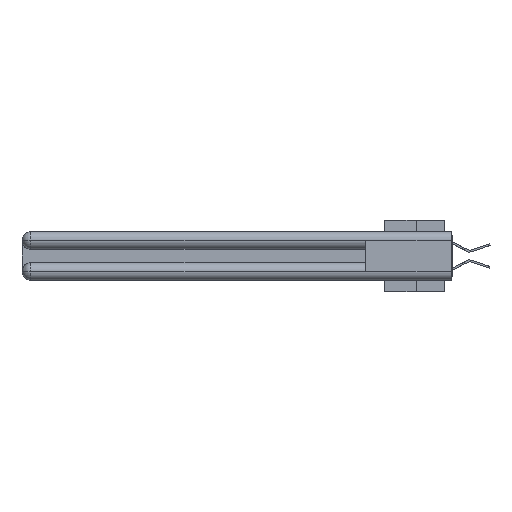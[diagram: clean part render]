
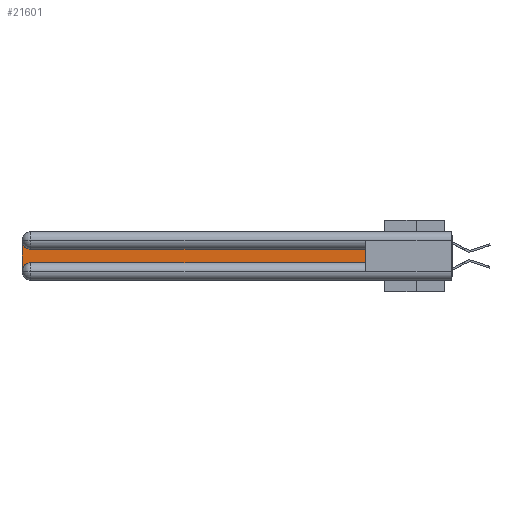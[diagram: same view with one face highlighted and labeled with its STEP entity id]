
A CAD part, left-side view. The second image highlights one B-rep face of the part: STEP entity #21601.
In plain terms, the highlighted planar face has unit normal (-1, 0, 0).
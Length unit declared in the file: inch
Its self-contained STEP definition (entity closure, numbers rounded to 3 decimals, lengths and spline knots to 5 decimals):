
#129 = VERTEX_POINT ( 'NONE', #13830 ) ;
#345 = AXIS2_PLACEMENT_3D ( 'NONE', #7179, #28323, #2479 ) ;
#801 = DIRECTION ( 'NONE',  ( 0., 1., 0. ) ) ;
#1193 = CIRCLE ( 'NONE', #16820, 0.06 ) ;
#2479 = DIRECTION ( 'NONE',  ( 0., 0., -1. ) ) ;
#4524 = DIRECTION ( 'NONE',  ( 0., -1., 0. ) ) ;
#5343 = CARTESIAN_POINT ( 'NONE',  ( 0.075, 0.6, -0.1225 ) ) ;
#5709 = CARTESIAN_POINT ( 'NONE',  ( 0.075, 2.94, -0.2775 ) ) ;
#5713 = EDGE_CURVE ( 'NONE', #21550, #12105, #23670, .T. ) ;
#5931 = CIRCLE ( 'NONE', #30431, 0.06 ) ;
#6310 = ORIENTED_EDGE ( 'NONE', *, *, #10745, .T. ) ;
#6891 = DIRECTION ( 'NONE',  ( 1., 0., 0. ) ) ;
#7179 = CARTESIAN_POINT ( 'NONE',  ( 0.075, 3., -0.1225 ) ) ;
#9151 = DIRECTION ( 'NONE',  ( 0., 0., -1. ) ) ;
#10745 = EDGE_CURVE ( 'NONE', #11620, #17671, #23314, .T. ) ;
#11353 = CARTESIAN_POINT ( 'NONE',  ( 0.075, 2.94, -0.0625 ) ) ;
#11408 = VECTOR ( 'NONE', #4524, 39.37008 ) ;
#11620 = VERTEX_POINT ( 'NONE', #21073 ) ;
#12105 = VERTEX_POINT ( 'NONE', #15975 ) ;
#12313 = CARTESIAN_POINT ( 'NONE',  ( 0.075, 2.94, -0.1225 ) ) ;
#12530 = CARTESIAN_POINT ( 'NONE',  ( 0.075, 3., -0.2775 ) ) ;
#13043 = DIRECTION ( 'NONE',  ( 1., 0., 0. ) ) ;
#13055 = ORIENTED_EDGE ( 'NONE', *, *, #21988, .T. ) ;
#13830 = CARTESIAN_POINT ( 'NONE',  ( 0.075, 2.94, -0.2175 ) ) ;
#14264 = VERTEX_POINT ( 'NONE', #12313 ) ;
#14452 = CARTESIAN_POINT ( 'NONE',  ( 0.075, 0.6, -0.2175 ) ) ;
#15285 = ORIENTED_EDGE ( 'NONE', *, *, #29850, .T. ) ;
#15975 = CARTESIAN_POINT ( 'NONE',  ( 0.075, 0.6, -0.1225 ) ) ;
#16073 = CARTESIAN_POINT ( 'NONE',  ( 0.075, 0.6, -0.2175 ) ) ;
#16195 = LINE ( 'NONE', #14452, #11408 ) ;
#16552 = EDGE_LOOP ( 'NONE', ( #30233, #16837, #6310, #13055, #15285, #23141 ) ) ;
#16721 = DIRECTION ( 'NONE',  ( 0., 0., -1. ) ) ;
#16820 = AXIS2_PLACEMENT_3D ( 'NONE', #5709, #13043, #17515 ) ;
#16837 = ORIENTED_EDGE ( 'NONE', *, *, #17209, .T. ) ;
#17209 = EDGE_CURVE ( 'NONE', #14264, #11620, #5931, .T. ) ;
#17515 = DIRECTION ( 'NONE',  ( 0., 0., -1. ) ) ;
#17671 = VERTEX_POINT ( 'NONE', #12530 ) ;
#18119 = DIRECTION ( 'NONE',  ( 0., 0., 1. ) ) ;
#18805 = CARTESIAN_POINT ( 'NONE',  ( 0.075, 3., -0.2175 ) ) ;
#19362 = FACE_OUTER_BOUND ( 'NONE', #16552, .T. ) ;
#21073 = CARTESIAN_POINT ( 'NONE',  ( 0.075, 3., -0.0625 ) ) ;
#21109 = VECTOR ( 'NONE', #16721, 39.37008 ) ;
#21550 = VERTEX_POINT ( 'NONE', #16073 ) ;
#21601 = ADVANCED_FACE ( 'NONE', ( #19362 ), #23677, .F. ) ;
#21988 = EDGE_CURVE ( 'NONE', #17671, #129, #1193, .T. ) ;
#23141 = ORIENTED_EDGE ( 'NONE', *, *, #5713, .T. ) ;
#23314 = LINE ( 'NONE', #18805, #21109 ) ;
#23670 = LINE ( 'NONE', #24706, #27355 ) ;
#23677 = PLANE ( 'NONE',  #345 ) ;
#24706 = CARTESIAN_POINT ( 'NONE',  ( 0.075, 0.6, -0.2175 ) ) ;
#25025 = EDGE_CURVE ( 'NONE', #12105, #14264, #25698, .T. ) ;
#25698 = LINE ( 'NONE', #5343, #26428 ) ;
#26428 = VECTOR ( 'NONE', #801, 39.37008 ) ;
#27355 = VECTOR ( 'NONE', #18119, 39.37008 ) ;
#28323 = DIRECTION ( 'NONE',  ( 1., 0., 0. ) ) ;
#29850 = EDGE_CURVE ( 'NONE', #129, #21550, #16195, .T. ) ;
#30233 = ORIENTED_EDGE ( 'NONE', *, *, #25025, .T. ) ;
#30431 = AXIS2_PLACEMENT_3D ( 'NONE', #11353, #6891, #9151 ) ;
